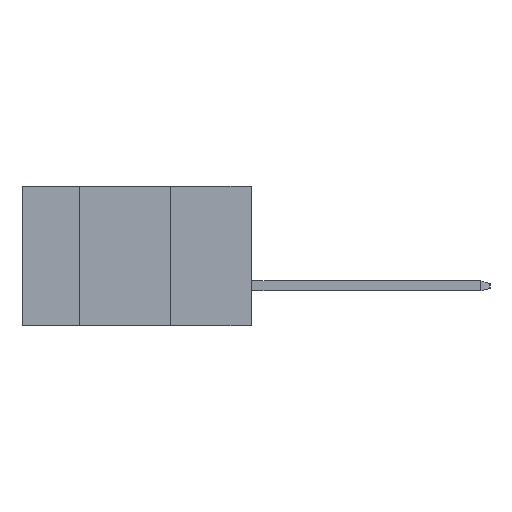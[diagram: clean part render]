
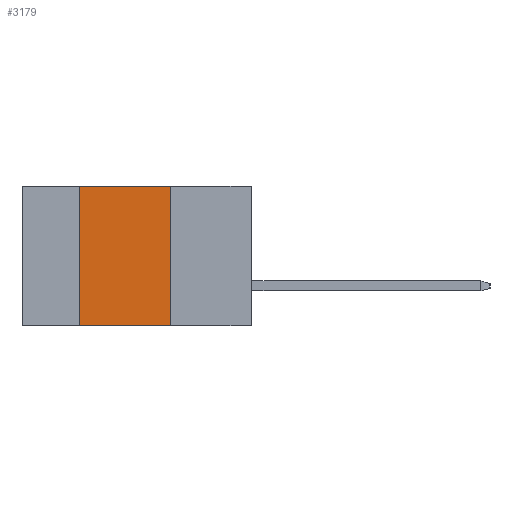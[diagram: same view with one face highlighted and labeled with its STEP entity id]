
A CAD part, left-side view. The second image highlights one B-rep face of the part: STEP entity #3179.
In plain terms, the highlighted planar face has unit normal (-1, 0, 0).
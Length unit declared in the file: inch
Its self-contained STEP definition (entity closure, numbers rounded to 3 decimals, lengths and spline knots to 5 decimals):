
#375 = DIRECTION ( 'NONE',  ( 0., 0., 1. ) ) ;
#685 = ORIENTED_EDGE ( 'NONE', *, *, #10502, .F. ) ;
#940 = CARTESIAN_POINT ( 'NONE',  ( 0., 0.72, 0. ) ) ;
#1034 = CARTESIAN_POINT ( 'NONE',  ( 0., 0.72, 0. ) ) ;
#2723 = VERTEX_POINT ( 'NONE', #11875 ) ;
#2751 = ORIENTED_EDGE ( 'NONE', *, *, #8714, .F. ) ;
#2760 = EDGE_CURVE ( 'NONE', #2903, #8245, #6467, .T. ) ;
#2861 = VECTOR ( 'NONE', #4486, 39.37008 ) ;
#2903 = VERTEX_POINT ( 'NONE', #5842 ) ;
#3030 = CARTESIAN_POINT ( 'NONE',  ( 0., 0.254, -0.437 ) ) ;
#3179 = ADVANCED_FACE ( 'NONE', ( #6518 ), #4691, .F. ) ;
#4034 = DIRECTION ( 'NONE',  ( 0., -1., 0. ) ) ;
#4377 = VECTOR ( 'NONE', #375, 39.37008 ) ;
#4486 = DIRECTION ( 'NONE',  ( 0., 0., -1. ) ) ;
#4569 = VERTEX_POINT ( 'NONE', #3030 ) ;
#4691 = PLANE ( 'NONE',  #8686 ) ;
#4743 = DIRECTION ( 'NONE',  ( 0., 0., -1. ) ) ;
#4936 = LINE ( 'NONE', #8642, #9638 ) ;
#5169 = CARTESIAN_POINT ( 'NONE',  ( 0., 0.254, -0.437 ) ) ;
#5180 = VECTOR ( 'NONE', #9978, 39.37008 ) ;
#5842 = CARTESIAN_POINT ( 'NONE',  ( 0., 0.54, 0. ) ) ;
#5919 = CARTESIAN_POINT ( 'NONE',  ( 0., 0.254, 0. ) ) ;
#6120 = EDGE_LOOP ( 'NONE', ( #685, #6513, #2751, #10960 ) ) ;
#6467 = LINE ( 'NONE', #940, #5180 ) ;
#6513 = ORIENTED_EDGE ( 'NONE', *, *, #2760, .F. ) ;
#6518 = FACE_OUTER_BOUND ( 'NONE', #6120, .T. ) ;
#6584 = DIRECTION ( 'NONE',  ( 1., 0., 0. ) ) ;
#8245 = VERTEX_POINT ( 'NONE', #5919 ) ;
#8642 = CARTESIAN_POINT ( 'NONE',  ( 0., 0.72, -0.437 ) ) ;
#8686 = AXIS2_PLACEMENT_3D ( 'NONE', #1034, #6584, #4743 ) ;
#8694 = LINE ( 'NONE', #11620, #4377 ) ;
#8714 = EDGE_CURVE ( 'NONE', #2723, #2903, #8694, .T. ) ;
#9102 = LINE ( 'NONE', #5169, #2861 ) ;
#9638 = VECTOR ( 'NONE', #4034, 39.37008 ) ;
#9978 = DIRECTION ( 'NONE',  ( 0., -1., 0. ) ) ;
#10502 = EDGE_CURVE ( 'NONE', #8245, #4569, #9102, .T. ) ;
#10960 = ORIENTED_EDGE ( 'NONE', *, *, #11709, .T. ) ;
#11620 = CARTESIAN_POINT ( 'NONE',  ( 0., 0.54, -0.437 ) ) ;
#11709 = EDGE_CURVE ( 'NONE', #2723, #4569, #4936, .T. ) ;
#11875 = CARTESIAN_POINT ( 'NONE',  ( 0., 0.54, -0.437 ) ) ;
